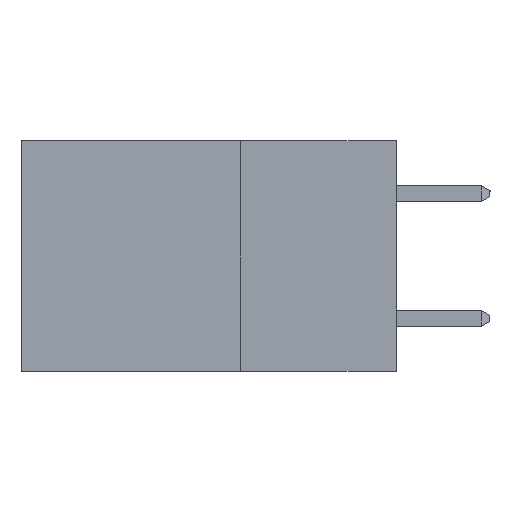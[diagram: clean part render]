
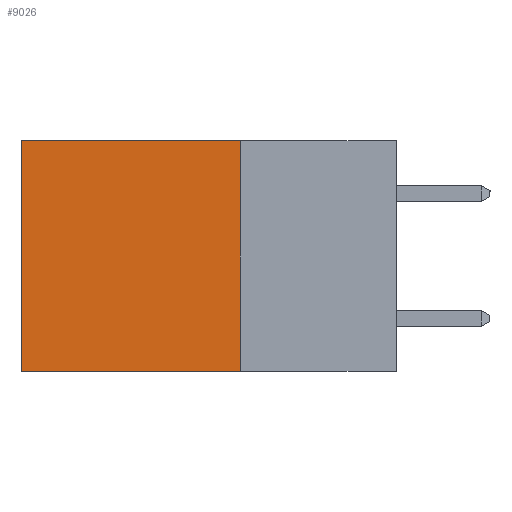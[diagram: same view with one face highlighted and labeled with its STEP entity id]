
A CAD part, left-side view. The second image highlights one B-rep face of the part: STEP entity #9026.
In plain terms, the highlighted planar face has unit normal (-1, 0, 0).
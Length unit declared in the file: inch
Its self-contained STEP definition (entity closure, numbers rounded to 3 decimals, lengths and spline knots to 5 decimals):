
#739 = VERTEX_POINT ( 'NONE', #9203 ) ;
#867 = EDGE_CURVE ( 'NONE', #9433, #739, #8666, .T. ) ;
#1473 = PLANE ( 'NONE',  #3643 ) ;
#2242 = LINE ( 'NONE', #8635, #5666 ) ;
#2937 = LINE ( 'NONE', #6987, #5491 ) ;
#3016 = EDGE_CURVE ( 'NONE', #9433, #9420, #8778, .T. ) ;
#3088 = CARTESIAN_POINT ( 'NONE',  ( 0.2615, 0.25, -0.37 ) ) ;
#3141 = DIRECTION ( 'NONE',  ( 0., 0., -1. ) ) ;
#3494 = ORIENTED_EDGE ( 'NONE', *, *, #867, .T. ) ;
#3643 = AXIS2_PLACEMENT_3D ( 'NONE', #3088, #7841, #4535 ) ;
#3956 = CARTESIAN_POINT ( 'NONE',  ( 0.2615, 0.25, -0.37 ) ) ;
#4535 = DIRECTION ( 'NONE',  ( 0., 0., -1. ) ) ;
#4633 = ORIENTED_EDGE ( 'NONE', *, *, #7316, .T. ) ;
#4741 = CARTESIAN_POINT ( 'NONE',  ( 0.2615, 0.25, 0. ) ) ;
#4776 = VECTOR ( 'NONE', #7897, 39.37008 ) ;
#4935 = VERTEX_POINT ( 'NONE', #9650 ) ;
#5384 = DIRECTION ( 'NONE',  ( 0., 1., 0. ) ) ;
#5491 = VECTOR ( 'NONE', #3141, 39.37008 ) ;
#5666 = VECTOR ( 'NONE', #5384, 39.37008 ) ;
#6371 = DIRECTION ( 'NONE',  ( 0., 0., -1. ) ) ;
#6707 = CARTESIAN_POINT ( 'NONE',  ( 0.2615, 0.25, -0.37 ) ) ;
#6814 = ORIENTED_EDGE ( 'NONE', *, *, #8193, .F. ) ;
#6987 = CARTESIAN_POINT ( 'NONE',  ( 0.2615, 0.6, -0.37 ) ) ;
#7316 = EDGE_CURVE ( 'NONE', #739, #4935, #2937, .T. ) ;
#7514 = CARTESIAN_POINT ( 'NONE',  ( 0.2615, 0.25, 0. ) ) ;
#7841 = DIRECTION ( 'NONE',  ( 1., 0., 0. ) ) ;
#7897 = DIRECTION ( 'NONE',  ( 0., 1., 0. ) ) ;
#8193 = EDGE_CURVE ( 'NONE', #9420, #4935, #2242, .T. ) ;
#8251 = EDGE_LOOP ( 'NONE', ( #4633, #6814, #8266, #3494 ) ) ;
#8266 = ORIENTED_EDGE ( 'NONE', *, *, #3016, .F. ) ;
#8473 = VECTOR ( 'NONE', #6371, 39.37008 ) ;
#8635 = CARTESIAN_POINT ( 'NONE',  ( 0.2615, 0.25, -0.37 ) ) ;
#8666 = LINE ( 'NONE', #4741, #4776 ) ;
#8778 = LINE ( 'NONE', #3956, #8473 ) ;
#9026 = ADVANCED_FACE ( 'NONE', ( #10003 ), #1473, .F. ) ;
#9203 = CARTESIAN_POINT ( 'NONE',  ( 0.2615, 0.6, 0. ) ) ;
#9420 = VERTEX_POINT ( 'NONE', #6707 ) ;
#9433 = VERTEX_POINT ( 'NONE', #7514 ) ;
#9650 = CARTESIAN_POINT ( 'NONE',  ( 0.2615, 0.6, -0.37 ) ) ;
#10003 = FACE_OUTER_BOUND ( 'NONE', #8251, .T. ) ;
